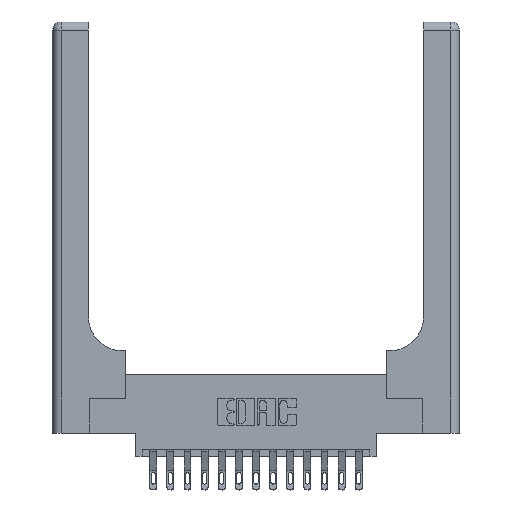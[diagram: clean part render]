
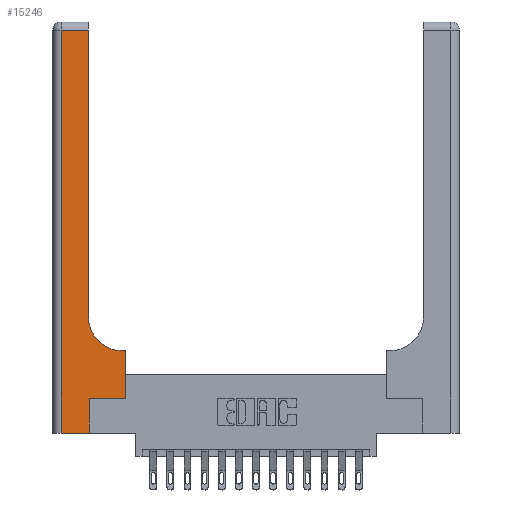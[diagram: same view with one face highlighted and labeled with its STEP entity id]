
A CAD part, top view. The second image highlights one B-rep face of the part: STEP entity #15246.
In plain terms, the highlighted planar face has unit normal (0, 0, 1).
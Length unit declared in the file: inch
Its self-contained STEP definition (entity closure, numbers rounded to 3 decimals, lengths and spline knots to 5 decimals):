
#558 = CARTESIAN_POINT ( 'NONE',  ( 0.26, 3., 0.37 ) ) ;
#908 = LINE ( 'NONE', #6602, #6529 ) ;
#1063 = CIRCLE ( 'NONE', #1973, 0.25 ) ;
#1245 = EDGE_CURVE ( 'NONE', #4911, #9829, #3958, .T. ) ;
#1567 = AXIS2_PLACEMENT_3D ( 'NONE', #4384, #9992, #15621 ) ;
#1973 = AXIS2_PLACEMENT_3D ( 'NONE', #15012, #11938, #12028 ) ;
#2121 = CARTESIAN_POINT ( 'NONE',  ( 0.528, 0.6, 0.37 ) ) ;
#2145 = ORIENTED_EDGE ( 'NONE', *, *, #8357, .T. ) ;
#2393 = VERTEX_POINT ( 'NONE', #16328 ) ;
#2501 = CARTESIAN_POINT ( 'NONE',  ( 0.06, 3., 0.37 ) ) ;
#2530 = EDGE_CURVE ( 'NONE', #4017, #10688, #6861, .T. ) ;
#2711 = VECTOR ( 'NONE', #5165, 39.37008 ) ;
#2901 = EDGE_LOOP ( 'NONE', ( #12847, #18327, #10856, #11214, #13331, #2145, #5370, #15714, #6747 ) ) ;
#3187 = CARTESIAN_POINT ( 'NONE',  ( 0., 0., 0.37 ) ) ;
#3334 = CARTESIAN_POINT ( 'NONE',  ( 0.528, 0.25, 0.37 ) ) ;
#3385 = LINE ( 'NONE', #9080, #4824 ) ;
#3958 = LINE ( 'NONE', #13875, #12564 ) ;
#4017 = VERTEX_POINT ( 'NONE', #4693 ) ;
#4277 = VECTOR ( 'NONE', #13757, 39.37008 ) ;
#4310 = DIRECTION ( 'NONE',  ( 1., 0., 0. ) ) ;
#4384 = CARTESIAN_POINT ( 'NONE',  ( 0., 3., 0.37 ) ) ;
#4675 = LINE ( 'NONE', #3187, #16238 ) ;
#4693 = CARTESIAN_POINT ( 'NONE',  ( 0.06, 2.94, 0.37 ) ) ;
#4824 = VECTOR ( 'NONE', #13395, 39.37008 ) ;
#4911 = VERTEX_POINT ( 'NONE', #3334 ) ;
#5165 = DIRECTION ( 'NONE',  ( 0., -1., 0. ) ) ;
#5173 = CARTESIAN_POINT ( 'NONE',  ( 0.265, 0., 0.37 ) ) ;
#5370 = ORIENTED_EDGE ( 'NONE', *, *, #1245, .T. ) ;
#6529 = VECTOR ( 'NONE', #12317, 39.37008 ) ;
#6602 = CARTESIAN_POINT ( 'NONE',  ( 0.265, 0.25, 0.37 ) ) ;
#6747 = ORIENTED_EDGE ( 'NONE', *, *, #11022, .T. ) ;
#6815 = EDGE_CURVE ( 'NONE', #9829, #10264, #8132, .T. ) ;
#6861 = LINE ( 'NONE', #2501, #2711 ) ;
#6900 = CARTESIAN_POINT ( 'NONE',  ( 0.26, 0.6, 0.37 ) ) ;
#7190 = PLANE ( 'NONE',  #1567 ) ;
#7541 = VERTEX_POINT ( 'NONE', #18252 ) ;
#8132 = LINE ( 'NONE', #6900, #9222 ) ;
#8174 = DIRECTION ( 'NONE',  ( 0., 1., 0. ) ) ;
#8357 = EDGE_CURVE ( 'NONE', #7541, #4911, #908, .T. ) ;
#8772 = VERTEX_POINT ( 'NONE', #13704 ) ;
#9080 = CARTESIAN_POINT ( 'NONE',  ( 0.265, 0., 0.37 ) ) ;
#9222 = VECTOR ( 'NONE', #16644, 39.37008 ) ;
#9801 = VERTEX_POINT ( 'NONE', #5173 ) ;
#9829 = VERTEX_POINT ( 'NONE', #2121 ) ;
#9992 = DIRECTION ( 'NONE',  ( 0., 0., -1. ) ) ;
#10264 = VERTEX_POINT ( 'NONE', #13587 ) ;
#10688 = VERTEX_POINT ( 'NONE', #13536 ) ;
#10738 = EDGE_CURVE ( 'NONE', #2393, #4017, #17749, .T. ) ;
#10856 = ORIENTED_EDGE ( 'NONE', *, *, #2530, .T. ) ;
#11020 = DIRECTION ( 'NONE',  ( -1., 0., 0. ) ) ;
#11022 = EDGE_CURVE ( 'NONE', #10264, #8772, #1063, .T. ) ;
#11214 = ORIENTED_EDGE ( 'NONE', *, *, #15995, .T. ) ;
#11938 = DIRECTION ( 'NONE',  ( 0., 0., -1. ) ) ;
#12028 = DIRECTION ( 'NONE',  ( 1., 0., 0. ) ) ;
#12237 = CARTESIAN_POINT ( 'NONE',  ( 0., 2.94, 0.37 ) ) ;
#12317 = DIRECTION ( 'NONE',  ( 1., 0., 0. ) ) ;
#12564 = VECTOR ( 'NONE', #8174, 39.37008 ) ;
#12802 = FACE_OUTER_BOUND ( 'NONE', #2901, .T. ) ;
#12847 = ORIENTED_EDGE ( 'NONE', *, *, #16127, .T. ) ;
#13331 = ORIENTED_EDGE ( 'NONE', *, *, #14633, .T. ) ;
#13395 = DIRECTION ( 'NONE',  ( 0., 1., 0. ) ) ;
#13536 = CARTESIAN_POINT ( 'NONE',  ( 0.06, 0., 0.37 ) ) ;
#13587 = CARTESIAN_POINT ( 'NONE',  ( 0.51, 0.6, 0.37 ) ) ;
#13668 = LINE ( 'NONE', #558, #4277 ) ;
#13704 = CARTESIAN_POINT ( 'NONE',  ( 0.26, 0.85, 0.37 ) ) ;
#13757 = DIRECTION ( 'NONE',  ( 0., 1., 0. ) ) ;
#13875 = CARTESIAN_POINT ( 'NONE',  ( 0.528, 0.25, 0.37 ) ) ;
#14633 = EDGE_CURVE ( 'NONE', #9801, #7541, #3385, .T. ) ;
#15012 = CARTESIAN_POINT ( 'NONE',  ( 0.51, 0.85, 0.37 ) ) ;
#15246 = ADVANCED_FACE ( 'NONE', ( #12802 ), #7190, .F. ) ;
#15621 = DIRECTION ( 'NONE',  ( -1., 0., 0. ) ) ;
#15714 = ORIENTED_EDGE ( 'NONE', *, *, #6815, .T. ) ;
#15995 = EDGE_CURVE ( 'NONE', #10688, #9801, #4675, .T. ) ;
#16127 = EDGE_CURVE ( 'NONE', #8772, #2393, #13668, .T. ) ;
#16238 = VECTOR ( 'NONE', #4310, 39.37008 ) ;
#16328 = CARTESIAN_POINT ( 'NONE',  ( 0.26, 2.94, 0.37 ) ) ;
#16644 = DIRECTION ( 'NONE',  ( -1., 0., 0. ) ) ;
#17749 = LINE ( 'NONE', #12237, #18225 ) ;
#18225 = VECTOR ( 'NONE', #11020, 39.37008 ) ;
#18252 = CARTESIAN_POINT ( 'NONE',  ( 0.265, 0.25, 0.37 ) ) ;
#18327 = ORIENTED_EDGE ( 'NONE', *, *, #10738, .T. ) ;
